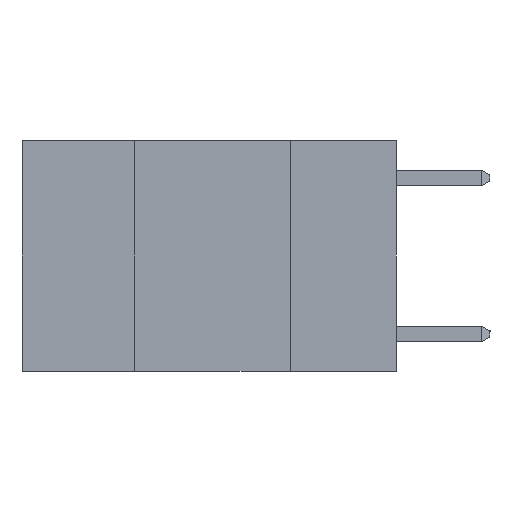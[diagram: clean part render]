
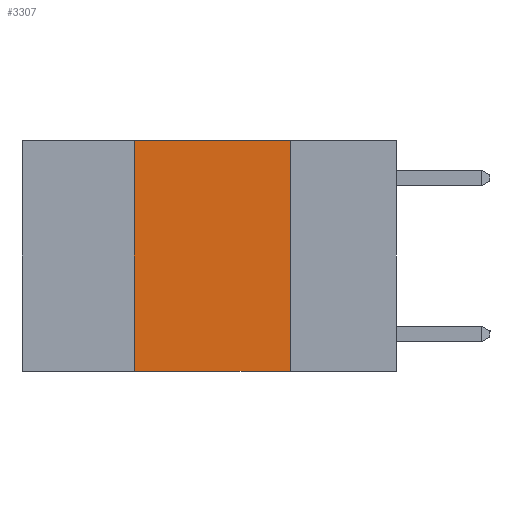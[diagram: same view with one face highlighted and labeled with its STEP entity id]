
A CAD part, left-side view. The second image highlights one B-rep face of the part: STEP entity #3307.
In plain terms, the highlighted planar face has unit normal (-1, 0, 0).
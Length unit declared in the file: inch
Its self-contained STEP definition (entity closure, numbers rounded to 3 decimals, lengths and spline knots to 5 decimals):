
#29 = DIRECTION ( 'NONE',  ( 0., 0., -1. ) ) ;
#367 = LINE ( 'NONE', #8311, #2694 ) ;
#592 = DIRECTION ( 'NONE',  ( 0., -1., 0. ) ) ;
#1136 = VECTOR ( 'NONE', #10997, 39.37008 ) ;
#1169 = ORIENTED_EDGE ( 'NONE', *, *, #2181, .F. ) ;
#1432 = ORIENTED_EDGE ( 'NONE', *, *, #3168, .T. ) ;
#1433 = EDGE_CURVE ( 'NONE', #3845, #4170, #10975, .T. ) ;
#2181 = EDGE_CURVE ( 'NONE', #4170, #7831, #10300, .T. ) ;
#2274 = CARTESIAN_POINT ( 'NONE',  ( 0., 0.17, 0. ) ) ;
#2694 = VECTOR ( 'NONE', #6072, 39.37008 ) ;
#2697 = AXIS2_PLACEMENT_3D ( 'NONE', #10551, #5948, #29 ) ;
#3071 = CARTESIAN_POINT ( 'NONE',  ( 0., 0.42, 0. ) ) ;
#3168 = EDGE_CURVE ( 'NONE', #3845, #4861, #8158, .T. ) ;
#3303 = CARTESIAN_POINT ( 'NONE',  ( 0., 0.42, -0.37 ) ) ;
#3307 = ADVANCED_FACE ( 'NONE', ( #10507 ), #5115, .F. ) ;
#3845 = VERTEX_POINT ( 'NONE', #3303 ) ;
#3950 = EDGE_LOOP ( 'NONE', ( #5488, #1169, #6041, #1432 ) ) ;
#4053 = EDGE_CURVE ( 'NONE', #7831, #4861, #367, .T. ) ;
#4170 = VERTEX_POINT ( 'NONE', #6407 ) ;
#4861 = VERTEX_POINT ( 'NONE', #5689 ) ;
#5115 = PLANE ( 'NONE',  #2697 ) ;
#5488 = ORIENTED_EDGE ( 'NONE', *, *, #4053, .F. ) ;
#5689 = CARTESIAN_POINT ( 'NONE',  ( 0., 0.17, -0.37 ) ) ;
#5948 = DIRECTION ( 'NONE',  ( 1., 0., 0. ) ) ;
#6041 = ORIENTED_EDGE ( 'NONE', *, *, #1433, .F. ) ;
#6072 = DIRECTION ( 'NONE',  ( 0., 0., -1. ) ) ;
#6407 = CARTESIAN_POINT ( 'NONE',  ( 0., 0.42, 0. ) ) ;
#7672 = DIRECTION ( 'NONE',  ( 0., 0., 1. ) ) ;
#7831 = VERTEX_POINT ( 'NONE', #2274 ) ;
#8158 = LINE ( 'NONE', #8804, #1136 ) ;
#8302 = VECTOR ( 'NONE', #592, 39.37008 ) ;
#8311 = CARTESIAN_POINT ( 'NONE',  ( 0., 0.17, 0. ) ) ;
#8804 = CARTESIAN_POINT ( 'NONE',  ( 0., 0.6, -0.37 ) ) ;
#8811 = VECTOR ( 'NONE', #7672, 39.37008 ) ;
#10256 = CARTESIAN_POINT ( 'NONE',  ( 0., 0.6, 0. ) ) ;
#10300 = LINE ( 'NONE', #10256, #8302 ) ;
#10507 = FACE_OUTER_BOUND ( 'NONE', #3950, .T. ) ;
#10551 = CARTESIAN_POINT ( 'NONE',  ( 0., 0.6, 0. ) ) ;
#10975 = LINE ( 'NONE', #3071, #8811 ) ;
#10997 = DIRECTION ( 'NONE',  ( 0., -1., 0. ) ) ;
